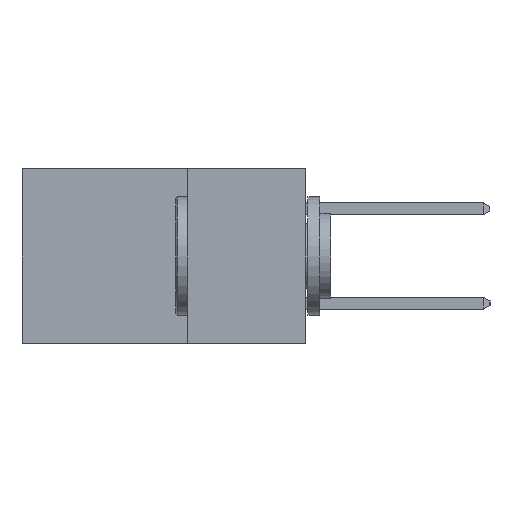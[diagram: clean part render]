
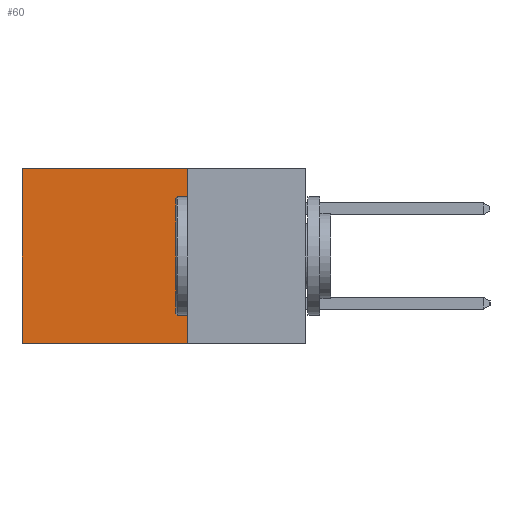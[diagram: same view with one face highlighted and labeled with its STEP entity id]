
A CAD part, left-side view. The second image highlights one B-rep face of the part: STEP entity #60.
In plain terms, the highlighted planar face has unit normal (-1, 0, 0).
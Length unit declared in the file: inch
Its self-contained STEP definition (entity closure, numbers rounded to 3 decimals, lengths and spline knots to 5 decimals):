
#60 = ADVANCED_FACE ( 'NONE', ( #3519 ), #2754, .F. ) ;
#66 = DIRECTION ( 'NONE',  ( 0., 0., -1. ) ) ;
#177 = VERTEX_POINT ( 'NONE', #7300 ) ;
#198 = VERTEX_POINT ( 'NONE', #9119 ) ;
#250 = LINE ( 'NONE', #1539, #7396 ) ;
#467 = ORIENTED_EDGE ( 'NONE', *, *, #6008, .T. ) ;
#1007 = DIRECTION ( 'NONE',  ( 1., 0., 0. ) ) ;
#1539 = CARTESIAN_POINT ( 'NONE',  ( 0.2615, 0.25, 0. ) ) ;
#2024 = CARTESIAN_POINT ( 'NONE',  ( 0.2615, 0.6, -0.37 ) ) ;
#2372 = CARTESIAN_POINT ( 'NONE',  ( 0.2615, 0.25, -0.37 ) ) ;
#2458 = CARTESIAN_POINT ( 'NONE',  ( 0.2615, 0.25, -0.37 ) ) ;
#2754 = PLANE ( 'NONE',  #4230 ) ;
#3070 = EDGE_CURVE ( 'NONE', #7445, #6733, #5627, .T. ) ;
#3244 = VECTOR ( 'NONE', #8283, 39.37008 ) ;
#3519 = FACE_OUTER_BOUND ( 'NONE', #8901, .T. ) ;
#4230 = AXIS2_PLACEMENT_3D ( 'NONE', #2458, #1007, #66 ) ;
#4359 = ORIENTED_EDGE ( 'NONE', *, *, #3070, .F. ) ;
#5533 = CARTESIAN_POINT ( 'NONE',  ( 0.2615, 0.6, -0.37 ) ) ;
#5627 = LINE ( 'NONE', #6779, #8967 ) ;
#5693 = DIRECTION ( 'NONE',  ( 0., 1., 0. ) ) ;
#5975 = DIRECTION ( 'NONE',  ( 0., 0., -1. ) ) ;
#6008 = EDGE_CURVE ( 'NONE', #198, #6733, #7017, .T. ) ;
#6066 = LINE ( 'NONE', #2372, #7841 ) ;
#6221 = ORIENTED_EDGE ( 'NONE', *, *, #6451, .F. ) ;
#6451 = EDGE_CURVE ( 'NONE', #177, #7445, #6066, .T. ) ;
#6733 = VERTEX_POINT ( 'NONE', #5533 ) ;
#6779 = CARTESIAN_POINT ( 'NONE',  ( 0.2615, 0.25, -0.37 ) ) ;
#7017 = LINE ( 'NONE', #2024, #3244 ) ;
#7300 = CARTESIAN_POINT ( 'NONE',  ( 0.2615, 0.25, 0. ) ) ;
#7351 = DIRECTION ( 'NONE',  ( 0., 1., 0. ) ) ;
#7396 = VECTOR ( 'NONE', #5693, 39.37008 ) ;
#7445 = VERTEX_POINT ( 'NONE', #8800 ) ;
#7841 = VECTOR ( 'NONE', #5975, 39.37008 ) ;
#7995 = ORIENTED_EDGE ( 'NONE', *, *, #8029, .T. ) ;
#8029 = EDGE_CURVE ( 'NONE', #177, #198, #250, .T. ) ;
#8283 = DIRECTION ( 'NONE',  ( 0., 0., -1. ) ) ;
#8800 = CARTESIAN_POINT ( 'NONE',  ( 0.2615, 0.25, -0.37 ) ) ;
#8901 = EDGE_LOOP ( 'NONE', ( #467, #4359, #6221, #7995 ) ) ;
#8967 = VECTOR ( 'NONE', #7351, 39.37008 ) ;
#9119 = CARTESIAN_POINT ( 'NONE',  ( 0.2615, 0.6, 0. ) ) ;
